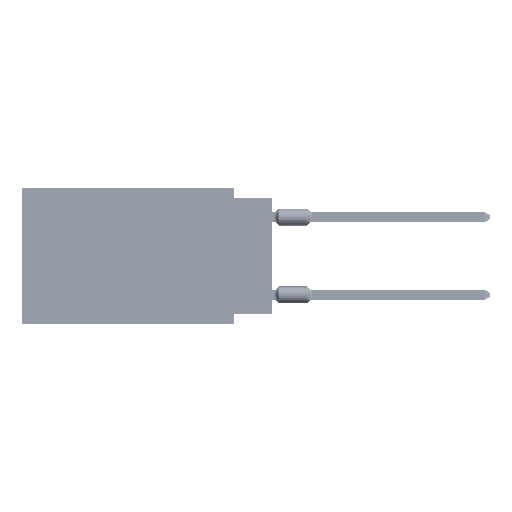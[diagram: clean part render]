
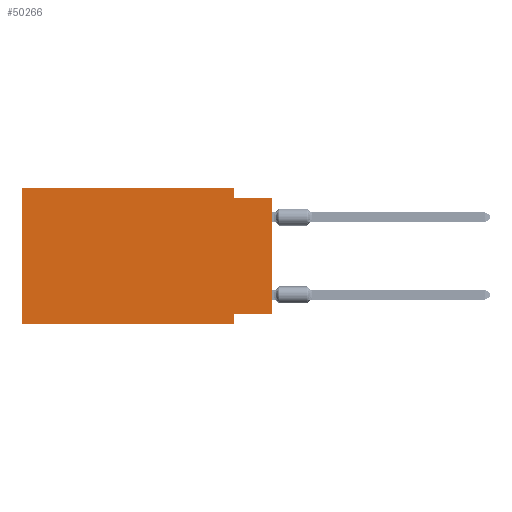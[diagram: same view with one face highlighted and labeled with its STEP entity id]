
A CAD part, left-side view. The second image highlights one B-rep face of the part: STEP entity #50266.
In plain terms, the highlighted planar face has unit normal (-1, 0, 0).
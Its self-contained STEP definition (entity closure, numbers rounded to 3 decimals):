
#1533 = CARTESIAN_POINT ( 'NONE',  ( 0., 2.54, -8.89 ) ) ;
#2068 = LINE ( 'NONE', #78427, #82391 ) ;
#6213 = CARTESIAN_POINT ( 'NONE',  ( 0., 2.54, 0. ) ) ;
#6448 = CARTESIAN_POINT ( 'NONE',  ( 0., 16.383, -8.89 ) ) ;
#7516 = CARTESIAN_POINT ( 'NONE',  ( 0., 16.383, 0. ) ) ;
#8283 = VECTOR ( 'NONE', #69046, 1000. ) ;
#10936 = LINE ( 'NONE', #1533, #8283 ) ;
#15320 = CARTESIAN_POINT ( 'NONE',  ( 0., 2.54, -8.255 ) ) ;
#15707 = VERTEX_POINT ( 'NONE', #26969 ) ;
#23169 = FACE_OUTER_BOUND ( 'NONE', #86590, .T. ) ;
#26969 = CARTESIAN_POINT ( 'NONE',  ( 0., 2.54, -0.635 ) ) ;
#27156 = VERTEX_POINT ( 'NONE', #35614 ) ;
#27240 = DIRECTION ( 'NONE',  ( 0., 0., 1. ) ) ;
#28471 = VERTEX_POINT ( 'NONE', #105181 ) ;
#31078 = CARTESIAN_POINT ( 'NONE',  ( 0., 2.54, 0. ) ) ;
#31469 = PLANE ( 'NONE',  #49685 ) ;
#33784 = ORIENTED_EDGE ( 'NONE', *, *, #97935, .T. ) ;
#35614 = CARTESIAN_POINT ( 'NONE',  ( 0., 0., -8.255 ) ) ;
#35670 = ORIENTED_EDGE ( 'NONE', *, *, #64796, .F. ) ;
#36825 = EDGE_CURVE ( 'NONE', #55756, #28471, #10936, .T. ) ;
#38287 = VECTOR ( 'NONE', #74331, 1000. ) ;
#38913 = LINE ( 'NONE', #98109, #98757 ) ;
#40552 = CARTESIAN_POINT ( 'NONE',  ( 0., 0., 0. ) ) ;
#45339 = CARTESIAN_POINT ( 'NONE',  ( 0., 0., -0.635 ) ) ;
#48470 = VERTEX_POINT ( 'NONE', #6213 ) ;
#49685 = AXIS2_PLACEMENT_3D ( 'NONE', #56918, #98418, #64684 ) ;
#50266 = ADVANCED_FACE ( 'NONE', ( #23169 ), #31469, .F. ) ;
#51466 = EDGE_CURVE ( 'NONE', #27156, #101464, #92560, .T. ) ;
#51657 = EDGE_CURVE ( 'NONE', #15707, #101464, #68735, .T. ) ;
#55756 = VERTEX_POINT ( 'NONE', #15320 ) ;
#56918 = CARTESIAN_POINT ( 'NONE',  ( 0., 16.383, 0. ) ) ;
#61340 = ORIENTED_EDGE ( 'NONE', *, *, #93856, .F. ) ;
#62417 = EDGE_CURVE ( 'NONE', #27156, #55756, #2068, .T. ) ;
#64684 = DIRECTION ( 'NONE',  ( 0., 0., -1. ) ) ;
#64790 = CARTESIAN_POINT ( 'NONE',  ( 0., 0., -0.635 ) ) ;
#64796 = EDGE_CURVE ( 'NONE', #98536, #48470, #38913, .T. ) ;
#68735 = LINE ( 'NONE', #45339, #103673 ) ;
#69046 = DIRECTION ( 'NONE',  ( 0., 0., -1. ) ) ;
#70342 = ORIENTED_EDGE ( 'NONE', *, *, #107894, .F. ) ;
#71456 = ORIENTED_EDGE ( 'NONE', *, *, #51657, .F. ) ;
#73146 = LINE ( 'NONE', #31078, #106315 ) ;
#74088 = LINE ( 'NONE', #107275, #82045 ) ;
#74331 = DIRECTION ( 'NONE',  ( 0., 0., 1. ) ) ;
#74613 = ORIENTED_EDGE ( 'NONE', *, *, #36825, .F. ) ;
#74818 = VERTEX_POINT ( 'NONE', #6448 ) ;
#77781 = ORIENTED_EDGE ( 'NONE', *, *, #51466, .T. ) ;
#78139 = LINE ( 'NONE', #86453, #108103 ) ;
#78427 = CARTESIAN_POINT ( 'NONE',  ( 0., 0., -8.255 ) ) ;
#78984 = DIRECTION ( 'NONE',  ( 0., 1., 0. ) ) ;
#82045 = VECTOR ( 'NONE', #89592, 1000. ) ;
#82391 = VECTOR ( 'NONE', #78984, 1000. ) ;
#86453 = CARTESIAN_POINT ( 'NONE',  ( 0., 16.383, 0. ) ) ;
#86590 = EDGE_LOOP ( 'NONE', ( #77781, #71456, #70342, #35670, #61340, #33784, #74613, #92527 ) ) ;
#89592 = DIRECTION ( 'NONE',  ( 0., -1., 0. ) ) ;
#92527 = ORIENTED_EDGE ( 'NONE', *, *, #62417, .F. ) ;
#92560 = LINE ( 'NONE', #40552, #38287 ) ;
#93856 = EDGE_CURVE ( 'NONE', #74818, #98536, #78139, .T. ) ;
#96246 = DIRECTION ( 'NONE',  ( 0., -1., 0. ) ) ;
#97935 = EDGE_CURVE ( 'NONE', #74818, #28471, #74088, .T. ) ;
#98109 = CARTESIAN_POINT ( 'NONE',  ( 0., 16.383, 0. ) ) ;
#98418 = DIRECTION ( 'NONE',  ( 1., 0., 0. ) ) ;
#98536 = VERTEX_POINT ( 'NONE', #7516 ) ;
#98578 = DIRECTION ( 'NONE',  ( 0., 0., -1. ) ) ;
#98757 = VECTOR ( 'NONE', #105333, 1000. ) ;
#101464 = VERTEX_POINT ( 'NONE', #64790 ) ;
#103673 = VECTOR ( 'NONE', #96246, 1000. ) ;
#105181 = CARTESIAN_POINT ( 'NONE',  ( 0., 2.54, -8.89 ) ) ;
#105333 = DIRECTION ( 'NONE',  ( 0., -1., 0. ) ) ;
#106315 = VECTOR ( 'NONE', #98578, 1000. ) ;
#107275 = CARTESIAN_POINT ( 'NONE',  ( 0., 16.383, -8.89 ) ) ;
#107894 = EDGE_CURVE ( 'NONE', #48470, #15707, #73146, .T. ) ;
#108103 = VECTOR ( 'NONE', #27240, 1000. ) ;
